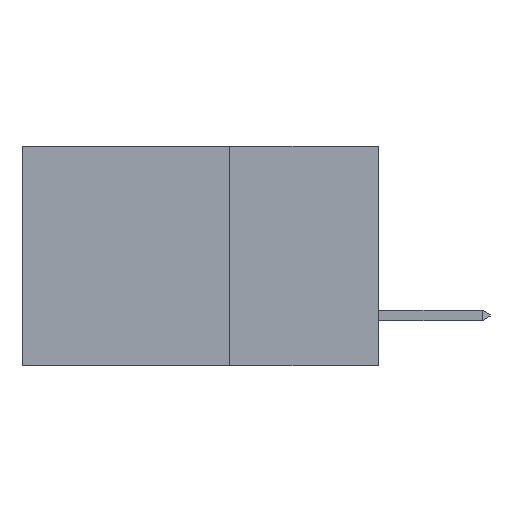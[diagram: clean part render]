
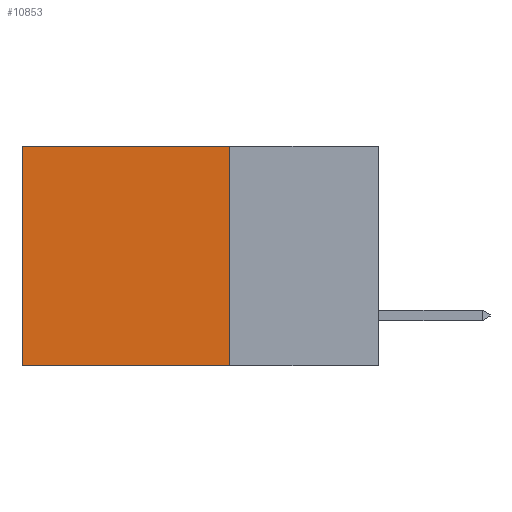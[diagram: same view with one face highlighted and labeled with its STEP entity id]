
A CAD part, left-side view. The second image highlights one B-rep face of the part: STEP entity #10853.
In plain terms, the highlighted planar face has unit normal (-1, 0, 0).
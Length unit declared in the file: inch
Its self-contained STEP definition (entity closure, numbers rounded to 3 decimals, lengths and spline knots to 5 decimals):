
#209 = DIRECTION ( 'NONE',  ( 0., 0., -1. ) ) ;
#527 = EDGE_CURVE ( 'NONE', #3207, #3632, #2544, .T. ) ;
#916 = DIRECTION ( 'NONE',  ( 0., 1., 0. ) ) ;
#1759 = ORIENTED_EDGE ( 'NONE', *, *, #4894, .F. ) ;
#1822 = CARTESIAN_POINT ( 'NONE',  ( 0.2615, 0.25, -0.37 ) ) ;
#1853 = ORIENTED_EDGE ( 'NONE', *, *, #6202, .T. ) ;
#1952 = ORIENTED_EDGE ( 'NONE', *, *, #527, .F. ) ;
#2032 = CARTESIAN_POINT ( 'NONE',  ( 0.2615, 0.6, -0.37 ) ) ;
#2118 = ORIENTED_EDGE ( 'NONE', *, *, #4388, .T. ) ;
#2250 = DIRECTION ( 'NONE',  ( 0., 0., -1. ) ) ;
#2435 = VECTOR ( 'NONE', #7593, 39.37008 ) ;
#2442 = CARTESIAN_POINT ( 'NONE',  ( 0.2615, 0.25, 0. ) ) ;
#2544 = LINE ( 'NONE', #10462, #9737 ) ;
#3207 = VERTEX_POINT ( 'NONE', #8982 ) ;
#3632 = VERTEX_POINT ( 'NONE', #8624 ) ;
#4388 = EDGE_CURVE ( 'NONE', #3207, #8046, #5450, .T. ) ;
#4843 = VECTOR ( 'NONE', #916, 39.37008 ) ;
#4894 = EDGE_CURVE ( 'NONE', #3632, #6578, #7519, .T. ) ;
#5109 = VECTOR ( 'NONE', #6259, 39.37008 ) ;
#5266 = CARTESIAN_POINT ( 'NONE',  ( 0.2615, 0.6, 0. ) ) ;
#5375 = PLANE ( 'NONE',  #7232 ) ;
#5450 = LINE ( 'NONE', #2442, #4843 ) ;
#6202 = EDGE_CURVE ( 'NONE', #8046, #6578, #10550, .T. ) ;
#6259 = DIRECTION ( 'NONE',  ( 0., 0., -1. ) ) ;
#6311 = DIRECTION ( 'NONE',  ( 1., 0., 0. ) ) ;
#6473 = FACE_OUTER_BOUND ( 'NONE', #8504, .T. ) ;
#6578 = VERTEX_POINT ( 'NONE', #2032 ) ;
#7232 = AXIS2_PLACEMENT_3D ( 'NONE', #9113, #6311, #209 ) ;
#7519 = LINE ( 'NONE', #1822, #2435 ) ;
#7593 = DIRECTION ( 'NONE',  ( 0., 1., 0. ) ) ;
#8046 = VERTEX_POINT ( 'NONE', #5266 ) ;
#8504 = EDGE_LOOP ( 'NONE', ( #1853, #1759, #1952, #2118 ) ) ;
#8624 = CARTESIAN_POINT ( 'NONE',  ( 0.2615, 0.25, -0.37 ) ) ;
#8982 = CARTESIAN_POINT ( 'NONE',  ( 0.2615, 0.25, 0. ) ) ;
#9113 = CARTESIAN_POINT ( 'NONE',  ( 0.2615, 0.25, -0.37 ) ) ;
#9737 = VECTOR ( 'NONE', #2250, 39.37008 ) ;
#10462 = CARTESIAN_POINT ( 'NONE',  ( 0.2615, 0.25, -0.37 ) ) ;
#10550 = LINE ( 'NONE', #11591, #5109 ) ;
#10853 = ADVANCED_FACE ( 'NONE', ( #6473 ), #5375, .F. ) ;
#11591 = CARTESIAN_POINT ( 'NONE',  ( 0.2615, 0.6, -0.37 ) ) ;
